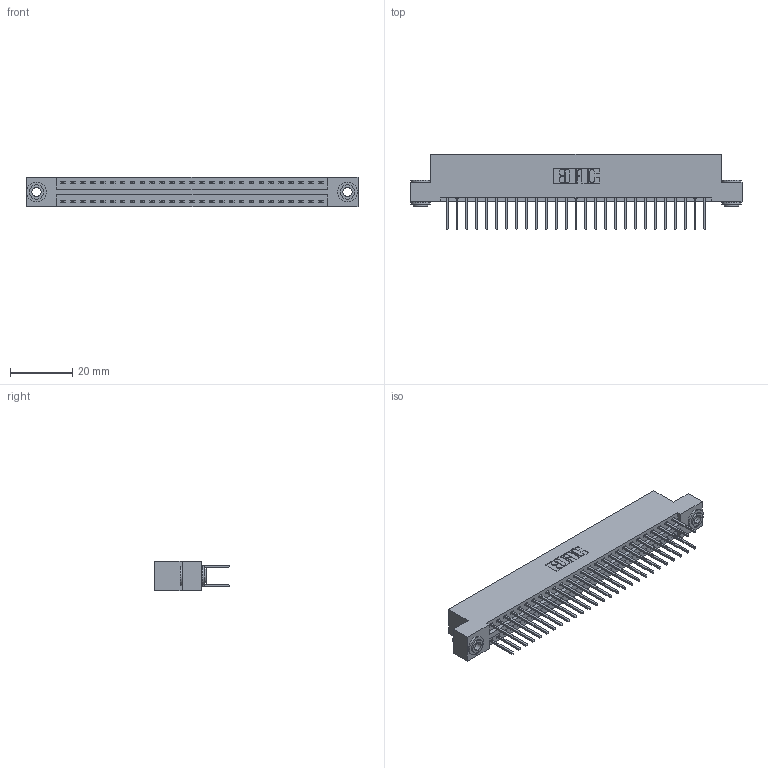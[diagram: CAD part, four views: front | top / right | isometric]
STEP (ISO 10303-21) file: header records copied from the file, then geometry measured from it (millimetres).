
FILE_DESCRIPTION (( 'STEP AP203' ), '1' );
FILE_NAME ('396-054-526-203.STEP', '2019-10-30T14:17:13', ( '' ), ( '' ), 'SwSTEP 2.0', 'SolidWorks 2016', '' );
FILE_SCHEMA (( 'CONFIG_CONTROL_DESIGN' ));
Length unit declared in the file: inch
Products named in the file (4): 346 Part_Flush Mounting Lugs - 0.156 Dia-TH; 345-292-001_345-293-126; 396-054-526-203; 345-250-002_345-250-002-102
Assembly tree (57 placements, depth 2):
  396-054-526-203
    346 Part_Flush Mounting Lugs - 0.156 Dia-TH
    345-292-001_345-293-126  x54
    345-250-002_345-250-002-102  x2
Bounding box: 106.3 x 24.13 x 9.4 mm (x, y, z)
Volume: 10356.9 mm3; surface area: 14611 mm2
Topology: 57 solids, 57 shells, 2968 faces, 8775 edges, 5774 vertices
Faces by surface type: plane 1976, cylinder 984, cone 8
Entity records: 20308 total; most frequent: CARTESIAN_POINT 3343, ORIENTED_EDGE 3270, DIRECTION 3029, EDGE_CURVE 1635, LINE 1371, VECTOR 1371, VERTEX_POINT 1086, AXIS2_PLACEMENT_3D 829
